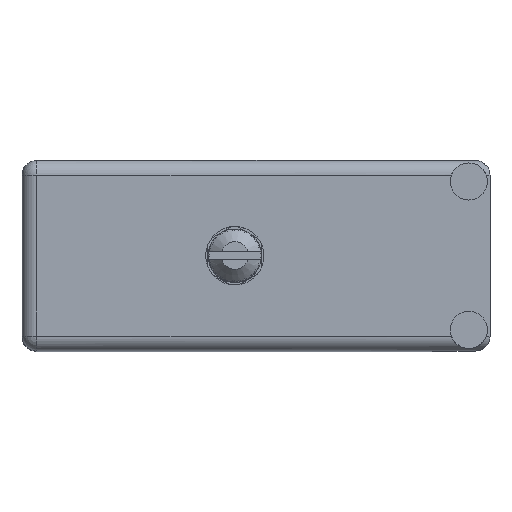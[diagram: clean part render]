
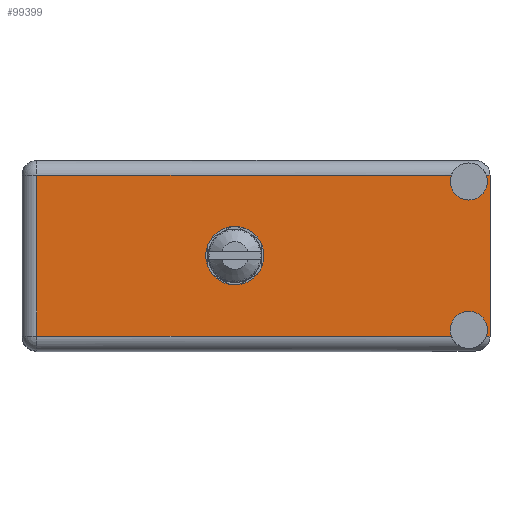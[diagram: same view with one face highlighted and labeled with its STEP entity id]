
A CAD part, top view. The second image highlights one B-rep face of the part: STEP entity #99399.
In plain terms, the highlighted face is planar.
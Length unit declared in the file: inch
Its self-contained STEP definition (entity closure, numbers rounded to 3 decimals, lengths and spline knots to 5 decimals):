
#650 = LINE ( 'NONE', #56362, #18882 ) ;
#1760 = DIRECTION ( 'NONE',  ( 0., 1., 0. ) ) ;
#3531 = VECTOR ( 'NONE', #71116, 39.37008 ) ;
#5125 = ORIENTED_EDGE ( 'NONE', *, *, #25210, .F. ) ;
#5427 = EDGE_CURVE ( 'NONE', #82439, #97750, #9654, .T. ) ;
#5970 = CARTESIAN_POINT ( 'NONE',  ( 1.004, 1.566, -0.587 ) ) ;
#6902 = CARTESIAN_POINT ( 'NONE',  ( 2.108, 1.566, -0.187 ) ) ;
#7053 = EDGE_CURVE ( 'NONE', #19251, #83985, #100653, .T. ) ;
#8925 = CARTESIAN_POINT ( 'NONE',  ( 2.208, 1.566, -0.07 ) ) ;
#9261 = DIRECTION ( 'NONE',  ( 0., 0., 1. ) ) ;
#9319 = DIRECTION ( 'NONE',  ( 1., 0., 0. ) ) ;
#9414 = FACE_BOUND ( 'NONE', #50570, .T. ) ;
#9654 = LINE ( 'NONE', #8925, #3531 ) ;
#9829 = DIRECTION ( 'NONE',  ( -1., 0., 0. ) ) ;
#10298 = AXIS2_PLACEMENT_3D ( 'NONE', #63697, #15880, #23676 ) ;
#11940 = DIRECTION ( 'NONE',  ( 0., 0., 1. ) ) ;
#12508 = CIRCLE ( 'NONE', #12809, 0.0875 ) ;
#12809 = AXIS2_PLACEMENT_3D ( 'NONE', #31692, #78589, #38494 ) ;
#13753 = CARTESIAN_POINT ( 'NONE',  ( 2.108, 1.566, -0.712 ) ) ;
#13761 = DIRECTION ( 'NONE',  ( 0., 1., 0. ) ) ;
#14465 = EDGE_CURVE ( 'NONE', #19251, #43907, #650, .T. ) ;
#15581 = CIRCLE ( 'NONE', #36779, 0.0875 ) ;
#15880 = DIRECTION ( 'NONE',  ( 0., 1., 0. ) ) ;
#18018 = CARTESIAN_POINT ( 'NONE',  ( 0., 1.566, -0.899 ) ) ;
#18882 = VECTOR ( 'NONE', #26799, 39.37008 ) ;
#19251 = VERTEX_POINT ( 'NONE', #30028 ) ;
#19313 = CARTESIAN_POINT ( 'NONE',  ( 2.108, 1.566, -0.0995 ) ) ;
#23676 = DIRECTION ( 'NONE',  ( 0., 0., 1. ) ) ;
#23940 = AXIS2_PLACEMENT_3D ( 'NONE', #63924, #1760, #9261 ) ;
#24299 = VERTEX_POINT ( 'NONE', #5970 ) ;
#25210 = EDGE_CURVE ( 'NONE', #24299, #75208, #68482, .T. ) ;
#26799 = DIRECTION ( 'NONE',  ( -1., 0., 0. ) ) ;
#26873 = CARTESIAN_POINT ( 'NONE',  ( 2.208, 1.566, 0. ) ) ;
#27790 = DIRECTION ( 'NONE',  ( 0., 0., 1. ) ) ;
#29512 = ORIENTED_EDGE ( 'NONE', *, *, #54083, .F. ) ;
#30028 = CARTESIAN_POINT ( 'NONE',  ( 2.02562, 1.566, -0.829 ) ) ;
#30044 = ORIENTED_EDGE ( 'NONE', *, *, #77710, .T. ) ;
#30777 = LINE ( 'NONE', #89652, #98780 ) ;
#31692 = CARTESIAN_POINT ( 'NONE',  ( 2.108, 1.566, -0.7995 ) ) ;
#32184 = ORIENTED_EDGE ( 'NONE', *, *, #44399, .F. ) ;
#32575 = DIRECTION ( 'NONE',  ( 0., 0., 1. ) ) ;
#33041 = CARTESIAN_POINT ( 'NONE',  ( 2.208, 1.566, -0.07 ) ) ;
#33693 = DIRECTION ( 'NONE',  ( 0., 1., 0. ) ) ;
#34615 = DIRECTION ( 'NONE',  ( 0., 0., 1. ) ) ;
#35695 = CARTESIAN_POINT ( 'NONE',  ( 2.19038, 1.566, -0.07 ) ) ;
#36342 = CIRCLE ( 'NONE', #10298, 0.1375 ) ;
#36412 = VECTOR ( 'NONE', #98154, 39.37008 ) ;
#36779 = AXIS2_PLACEMENT_3D ( 'NONE', #19313, #66149, #27790 ) ;
#38494 = DIRECTION ( 'NONE',  ( 0., 0., 1. ) ) ;
#41916 = AXIS2_PLACEMENT_3D ( 'NONE', #80276, #33693, #11940 ) ;
#42390 = ORIENTED_EDGE ( 'NONE', *, *, #5427, .T. ) ;
#43521 = VERTEX_POINT ( 'NONE', #46788 ) ;
#43907 = VERTEX_POINT ( 'NONE', #83790 ) ;
#44399 = EDGE_CURVE ( 'NONE', #82439, #100237, #67963, .T. ) ;
#44757 = CARTESIAN_POINT ( 'NONE',  ( 2.19038, 1.566, -0.829 ) ) ;
#45364 = CARTESIAN_POINT ( 'NONE',  ( 2.108, 1.566, -0.0995 ) ) ;
#45872 = ORIENTED_EDGE ( 'NONE', *, *, #86590, .T. ) ;
#46788 = CARTESIAN_POINT ( 'NONE',  ( 2.208, 1.566, -0.829 ) ) ;
#50570 = EDGE_LOOP ( 'NONE', ( #93034, #5125 ) ) ;
#53394 = LINE ( 'NONE', #26873, #36412 ) ;
#53448 = LINE ( 'NONE', #33041, #55864 ) ;
#54083 = EDGE_CURVE ( 'NONE', #43521, #97750, #53394, .T. ) ;
#55702 = DIRECTION ( 'NONE',  ( 0., 1., 0. ) ) ;
#55864 = VECTOR ( 'NONE', #9319, 39.37008 ) ;
#56362 = CARTESIAN_POINT ( 'NONE',  ( 0., 1.566, -0.829 ) ) ;
#57134 = ORIENTED_EDGE ( 'NONE', *, *, #58784, .F. ) ;
#57915 = AXIS2_PLACEMENT_3D ( 'NONE', #45364, #13761, #68128 ) ;
#58216 = CARTESIAN_POINT ( 'NONE',  ( 1.004, 1.566, -0.312 ) ) ;
#58784 = EDGE_CURVE ( 'NONE', #100237, #73842, #15581, .T. ) ;
#59420 = VERTEX_POINT ( 'NONE', #85365 ) ;
#62122 = EDGE_LOOP ( 'NONE', ( #30044, #57134, #32184, #42390, #29512, #68292, #81560, #100555, #85800, #45872 ) ) ;
#63697 = CARTESIAN_POINT ( 'NONE',  ( 1.004, 1.566, -0.4495 ) ) ;
#63924 = CARTESIAN_POINT ( 'NONE',  ( 1.004, 1.566, -0.4495 ) ) ;
#64924 = EDGE_CURVE ( 'NONE', #43521, #87863, #94889, .T. ) ;
#66149 = DIRECTION ( 'NONE',  ( 0., 1., 0. ) ) ;
#67963 = CIRCLE ( 'NONE', #57915, 0.0875 ) ;
#68128 = DIRECTION ( 'NONE',  ( 0., 0., 1. ) ) ;
#68292 = ORIENTED_EDGE ( 'NONE', *, *, #64924, .T. ) ;
#68482 = CIRCLE ( 'NONE', #23940, 0.1375 ) ;
#69816 = EDGE_CURVE ( 'NONE', #75208, #24299, #36342, .T. ) ;
#71116 = DIRECTION ( 'NONE',  ( 1., 0., 0. ) ) ;
#71597 = AXIS2_PLACEMENT_3D ( 'NONE', #18018, #55702, #32575 ) ;
#71689 = PLANE ( 'NONE',  #71597 ) ;
#73842 = VERTEX_POINT ( 'NONE', #97851 ) ;
#75208 = VERTEX_POINT ( 'NONE', #58216 ) ;
#77710 = EDGE_CURVE ( 'NONE', #59420, #73842, #53448, .T. ) ;
#78589 = DIRECTION ( 'NONE',  ( 0., 1., 0. ) ) ;
#78723 = FACE_OUTER_BOUND ( 'NONE', #62122, .T. ) ;
#79142 = CARTESIAN_POINT ( 'NONE',  ( 0., 1.566, -0.829 ) ) ;
#80276 = CARTESIAN_POINT ( 'NONE',  ( 2.108, 1.566, -0.7995 ) ) ;
#81560 = ORIENTED_EDGE ( 'NONE', *, *, #84270, .F. ) ;
#82439 = VERTEX_POINT ( 'NONE', #35695 ) ;
#82873 = VECTOR ( 'NONE', #9829, 39.37008 ) ;
#83790 = CARTESIAN_POINT ( 'NONE',  ( 0.07, 1.566, -0.829 ) ) ;
#83985 = VERTEX_POINT ( 'NONE', #13753 ) ;
#84270 = EDGE_CURVE ( 'NONE', #83985, #87863, #12508, .T. ) ;
#85365 = CARTESIAN_POINT ( 'NONE',  ( 0.07, 1.566, -0.07 ) ) ;
#85800 = ORIENTED_EDGE ( 'NONE', *, *, #14465, .T. ) ;
#86590 = EDGE_CURVE ( 'NONE', #43907, #59420, #30777, .T. ) ;
#87863 = VERTEX_POINT ( 'NONE', #44757 ) ;
#89652 = CARTESIAN_POINT ( 'NONE',  ( 0.07, 1.566, -0.899 ) ) ;
#93034 = ORIENTED_EDGE ( 'NONE', *, *, #69816, .F. ) ;
#94889 = LINE ( 'NONE', #79142, #82873 ) ;
#97750 = VERTEX_POINT ( 'NONE', #98460 ) ;
#97851 = CARTESIAN_POINT ( 'NONE',  ( 2.02562, 1.566, -0.07 ) ) ;
#98154 = DIRECTION ( 'NONE',  ( 0., 0., 1. ) ) ;
#98460 = CARTESIAN_POINT ( 'NONE',  ( 2.208, 1.566, -0.07 ) ) ;
#98780 = VECTOR ( 'NONE', #34615, 39.37008 ) ;
#99399 = ADVANCED_FACE ( 'NONE', ( #9414, #78723 ), #71689, .T. ) ;
#100237 = VERTEX_POINT ( 'NONE', #6902 ) ;
#100555 = ORIENTED_EDGE ( 'NONE', *, *, #7053, .F. ) ;
#100653 = CIRCLE ( 'NONE', #41916, 0.0875 ) ;
